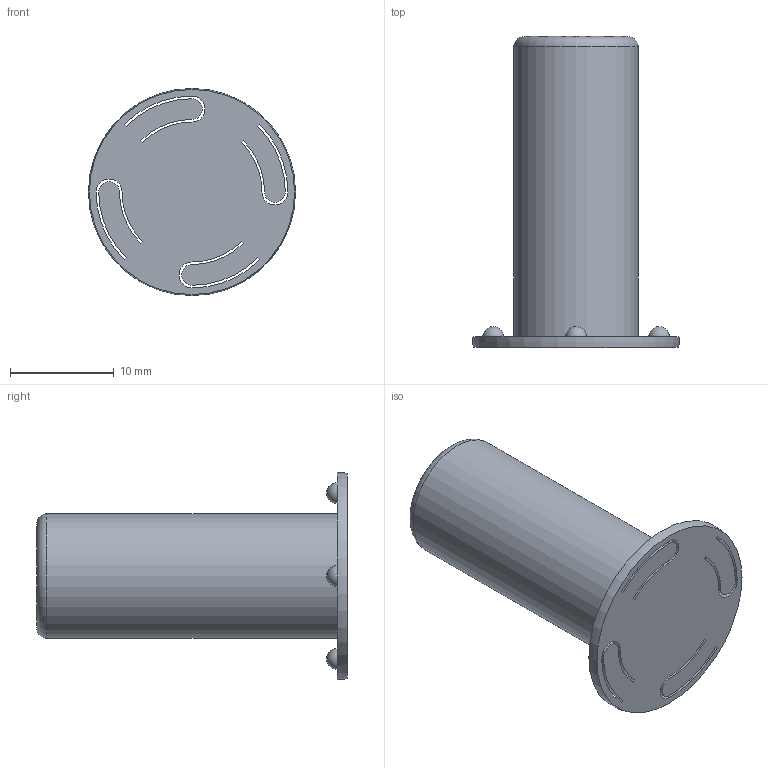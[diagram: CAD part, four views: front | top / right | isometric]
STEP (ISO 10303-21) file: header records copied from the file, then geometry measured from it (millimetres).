
FILE_DESCRIPTION (( 'STEP AP214' ), '1' );
FILE_NAME ('Bipod_Peg_Part_1_V2.step', '2016-01-25T18:17:13', ( 'WarFairy' ), ( '' ), 'SwSTEP 2.0', 'SolidWorks 2015', '' );
FILE_SCHEMA (( 'AUTOMOTIVE_DESIGN' ));
Length unit declared in the file: millimetre
Products named in the file (1): Bipod_Peg_Part_1_V2
Bounding box: 20 x 30 x 20 mm (x, y, z)
Volume: 3576.4 mm3; surface area: 1872.9 mm2
Topology: 1 solids, 1 shells, 42 faces, 118 edges, 75 vertices
Faces by surface type: cylinder 25, plane 11, sphere 4, torus 2
Full cylindrical faces by diameter (mm): 12 x1
Entity records: 1332 total; most frequent: DIRECTION 248, CARTESIAN_POINT 217, ORIENTED_EDGE 210, EDGE_CURVE 105, AXIS2_PLACEMENT_3D 100, VERTEX_POINT 69, CIRCLE 57, EDGE_LOOP 54
